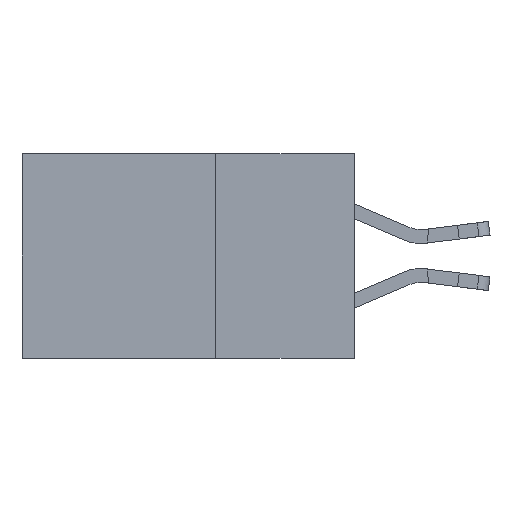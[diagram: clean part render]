
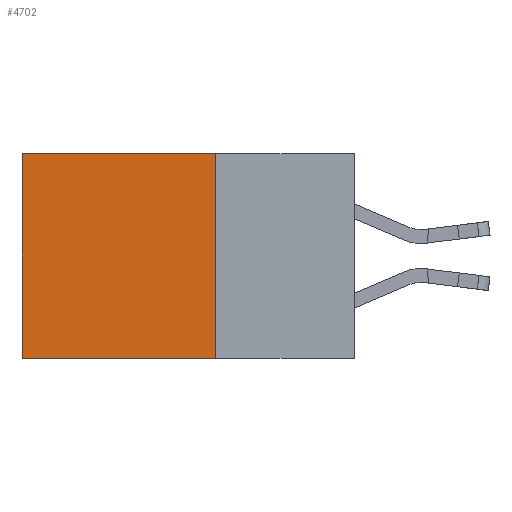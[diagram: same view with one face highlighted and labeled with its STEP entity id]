
A CAD part, left-side view. The second image highlights one B-rep face of the part: STEP entity #4702.
In plain terms, the highlighted planar face has unit normal (-1, 0, 0).
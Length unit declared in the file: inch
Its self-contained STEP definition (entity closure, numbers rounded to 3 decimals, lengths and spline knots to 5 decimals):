
#842 = CARTESIAN_POINT ( 'NONE',  ( 0.298, 0.6, 0. ) ) ;
#1039 = CARTESIAN_POINT ( 'NONE',  ( 0.298, 0.6, 0. ) ) ;
#1202 = DIRECTION ( 'NONE',  ( 0., 0., -1. ) ) ;
#1394 = ORIENTED_EDGE ( 'NONE', *, *, #8529, .F. ) ;
#2686 = PLANE ( 'NONE',  #3847 ) ;
#2858 = VERTEX_POINT ( 'NONE', #2966 ) ;
#2917 = CARTESIAN_POINT ( 'NONE',  ( 0.298, 0.25, 0. ) ) ;
#2966 = CARTESIAN_POINT ( 'NONE',  ( 0.298, 0.25, -0.37 ) ) ;
#3060 = DIRECTION ( 'NONE',  ( 0., 1., 0. ) ) ;
#3402 = FACE_OUTER_BOUND ( 'NONE', #10698, .T. ) ;
#3781 = VERTEX_POINT ( 'NONE', #1039 ) ;
#3847 = AXIS2_PLACEMENT_3D ( 'NONE', #5768, #7479, #11518 ) ;
#4126 = CARTESIAN_POINT ( 'NONE',  ( 0.298, 0.25, 0. ) ) ;
#4269 = VERTEX_POINT ( 'NONE', #9423 ) ;
#4702 = ADVANCED_FACE ( 'NONE', ( #3402 ), #2686, .F. ) ;
#4961 = LINE ( 'NONE', #842, #7575 ) ;
#5703 = EDGE_CURVE ( 'NONE', #2858, #4269, #10477, .T. ) ;
#5768 = CARTESIAN_POINT ( 'NONE',  ( 0.298, 0.25, 0. ) ) ;
#5771 = LINE ( 'NONE', #7167, #10709 ) ;
#5969 = EDGE_CURVE ( 'NONE', #10580, #3781, #10330, .T. ) ;
#7167 = CARTESIAN_POINT ( 'NONE',  ( 0.298, 0.25, 0. ) ) ;
#7316 = DIRECTION ( 'NONE',  ( 0., 1., 0. ) ) ;
#7479 = DIRECTION ( 'NONE',  ( 1., 0., 0. ) ) ;
#7555 = CARTESIAN_POINT ( 'NONE',  ( 0.298, 0.25, -0.37 ) ) ;
#7575 = VECTOR ( 'NONE', #9825, 39.37008 ) ;
#7786 = VECTOR ( 'NONE', #7316, 39.37008 ) ;
#8335 = EDGE_CURVE ( 'NONE', #3781, #4269, #4961, .T. ) ;
#8529 = EDGE_CURVE ( 'NONE', #10580, #2858, #5771, .T. ) ;
#9046 = ORIENTED_EDGE ( 'NONE', *, *, #5703, .F. ) ;
#9371 = ORIENTED_EDGE ( 'NONE', *, *, #5969, .T. ) ;
#9423 = CARTESIAN_POINT ( 'NONE',  ( 0.298, 0.6, -0.37 ) ) ;
#9825 = DIRECTION ( 'NONE',  ( 0., 0., -1. ) ) ;
#10330 = LINE ( 'NONE', #4126, #12860 ) ;
#10477 = LINE ( 'NONE', #7555, #7786 ) ;
#10580 = VERTEX_POINT ( 'NONE', #2917 ) ;
#10698 = EDGE_LOOP ( 'NONE', ( #11359, #9046, #1394, #9371 ) ) ;
#10709 = VECTOR ( 'NONE', #1202, 39.37008 ) ;
#11359 = ORIENTED_EDGE ( 'NONE', *, *, #8335, .T. ) ;
#11518 = DIRECTION ( 'NONE',  ( 0., 0., -1. ) ) ;
#12860 = VECTOR ( 'NONE', #3060, 39.37008 ) ;
